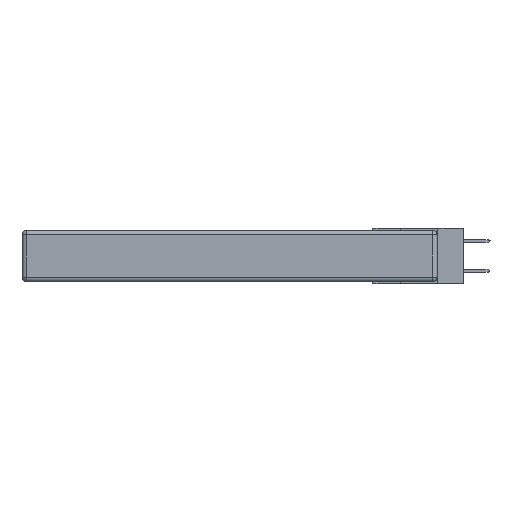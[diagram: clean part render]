
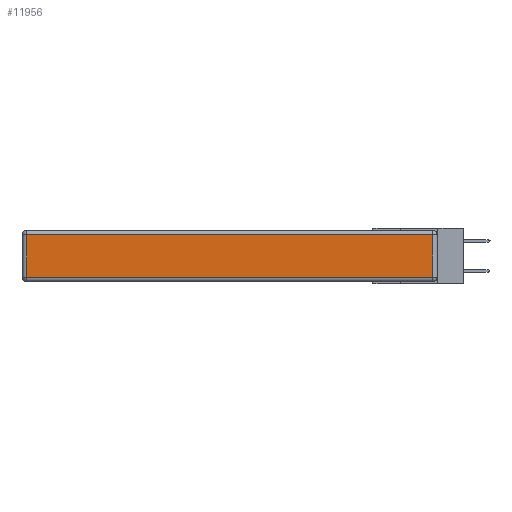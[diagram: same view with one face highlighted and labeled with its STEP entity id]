
A CAD part, left-side view. The second image highlights one B-rep face of the part: STEP entity #11956.
In plain terms, the highlighted planar face has unit normal (-1, 0, 0).
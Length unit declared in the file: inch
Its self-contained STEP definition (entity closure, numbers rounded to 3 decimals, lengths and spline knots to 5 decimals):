
#288 = VECTOR ( 'NONE', #25183, 39.37008 ) ;
#608 = FACE_OUTER_BOUND ( 'NONE', #3119, .T. ) ;
#714 = VECTOR ( 'NONE', #25438, 39.37008 ) ;
#1619 = EDGE_CURVE ( 'NONE', #6783, #3681, #16676, .T. ) ;
#1908 = EDGE_CURVE ( 'NONE', #3681, #2967, #18499, .T. ) ;
#2967 = VERTEX_POINT ( 'NONE', #23451 ) ;
#3119 = EDGE_LOOP ( 'NONE', ( #4853, #14601, #20111, #14696 ) ) ;
#3581 = LINE ( 'NONE', #21472, #18883 ) ;
#3681 = VERTEX_POINT ( 'NONE', #9607 ) ;
#4853 = ORIENTED_EDGE ( 'NONE', *, *, #1619, .T. ) ;
#5320 = DIRECTION ( 'NONE',  ( 0., 0., -1. ) ) ;
#5537 = CARTESIAN_POINT ( 'NONE',  ( 0., 0., -0.343 ) ) ;
#5567 = LINE ( 'NONE', #11274, #288 ) ;
#6590 = EDGE_CURVE ( 'NONE', #17561, #6783, #3581, .T. ) ;
#6783 = VERTEX_POINT ( 'NONE', #23418 ) ;
#7178 = AXIS2_PLACEMENT_3D ( 'NONE', #5537, #15221, #13223 ) ;
#7244 = PLANE ( 'NONE',  #7178 ) ;
#9304 = EDGE_CURVE ( 'NONE', #2967, #17561, #5567, .T. ) ;
#9607 = CARTESIAN_POINT ( 'NONE',  ( 0., 0.03, -0.313 ) ) ;
#11274 = CARTESIAN_POINT ( 'NONE',  ( 0., 2.75, -0.03 ) ) ;
#11956 = ADVANCED_FACE ( 'NONE', ( #608 ), #7244, .T. ) ;
#13223 = DIRECTION ( 'NONE',  ( 0., 0., 1. ) ) ;
#14124 = CARTESIAN_POINT ( 'NONE',  ( 0., 2.72, -0.03 ) ) ;
#14601 = ORIENTED_EDGE ( 'NONE', *, *, #1908, .T. ) ;
#14696 = ORIENTED_EDGE ( 'NONE', *, *, #6590, .T. ) ;
#15221 = DIRECTION ( 'NONE',  ( -1., 0., 0. ) ) ;
#16676 = LINE ( 'NONE', #25621, #714 ) ;
#17561 = VERTEX_POINT ( 'NONE', #14124 ) ;
#18499 = LINE ( 'NONE', #24974, #19095 ) ;
#18883 = VECTOR ( 'NONE', #5320, 39.37008 ) ;
#19095 = VECTOR ( 'NONE', #20716, 39.37008 ) ;
#20111 = ORIENTED_EDGE ( 'NONE', *, *, #9304, .T. ) ;
#20716 = DIRECTION ( 'NONE',  ( 0., 0., 1. ) ) ;
#21472 = CARTESIAN_POINT ( 'NONE',  ( 0., 2.72, -0.343 ) ) ;
#23418 = CARTESIAN_POINT ( 'NONE',  ( 0., 2.72, -0.313 ) ) ;
#23451 = CARTESIAN_POINT ( 'NONE',  ( 0., 0.03, -0.03 ) ) ;
#24974 = CARTESIAN_POINT ( 'NONE',  ( 0., 0.03, -0.343 ) ) ;
#25183 = DIRECTION ( 'NONE',  ( 0., 1., 0. ) ) ;
#25438 = DIRECTION ( 'NONE',  ( 0., -1., 0. ) ) ;
#25621 = CARTESIAN_POINT ( 'NONE',  ( 0., 0., -0.313 ) ) ;
